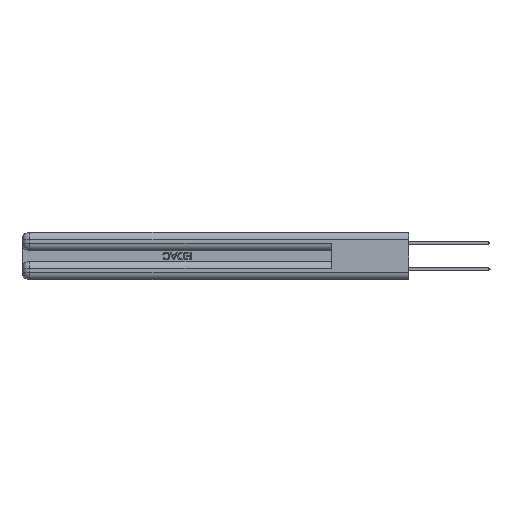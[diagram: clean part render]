
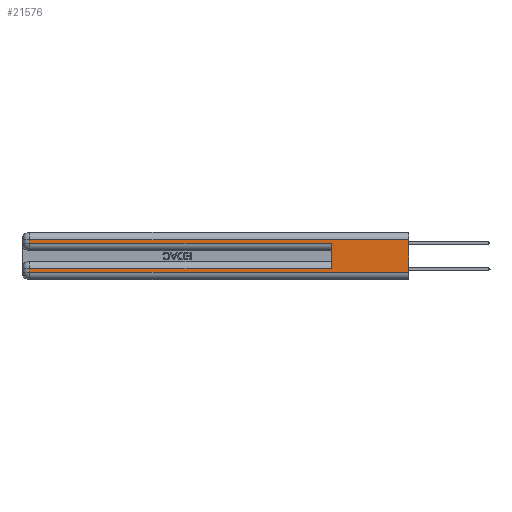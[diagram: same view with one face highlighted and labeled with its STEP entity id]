
A CAD part, left-side view. The second image highlights one B-rep face of the part: STEP entity #21576.
In plain terms, the highlighted planar face has unit normal (-1, 0, 0).
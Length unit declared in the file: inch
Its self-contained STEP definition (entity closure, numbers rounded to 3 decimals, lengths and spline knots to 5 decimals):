
#210 = AXIS2_PLACEMENT_3D ( 'NONE', #48010, #25254, #2502 ) ;
#254 = LINE ( 'NONE', #2577, #39509 ) ;
#1376 = LINE ( 'NONE', #38945, #48323 ) ;
#2502 = DIRECTION ( 'NONE',  ( 0., 0., -1. ) ) ;
#2577 = CARTESIAN_POINT ( 'NONE',  ( 0., 0., 0.31 ) ) ;
#2820 = CARTESIAN_POINT ( 'NONE',  ( 0., 2.94, 0.06 ) ) ;
#3358 = DIRECTION ( 'NONE',  ( 0., 0., 1. ) ) ;
#3640 = CARTESIAN_POINT ( 'NONE',  ( 0., 2.94, 0.085 ) ) ;
#4225 = VECTOR ( 'NONE', #24502, 39.37008 ) ;
#4384 = CARTESIAN_POINT ( 'NONE',  ( 0., 0., 0.31 ) ) ;
#7196 = EDGE_CURVE ( 'NONE', #16572, #26620, #23655, .T. ) ;
#8364 = CARTESIAN_POINT ( 'NONE',  ( 0., 2.94, 0.37 ) ) ;
#9181 = VECTOR ( 'NONE', #3358, 39.37008 ) ;
#9287 = ORIENTED_EDGE ( 'NONE', *, *, #15820, .F. ) ;
#10063 = DIRECTION ( 'NONE',  ( 0., 1., 0. ) ) ;
#10263 = EDGE_CURVE ( 'NONE', #26580, #30235, #36626, .T. ) ;
#11100 = ORIENTED_EDGE ( 'NONE', *, *, #7196, .T. ) ;
#12165 = CARTESIAN_POINT ( 'NONE',  ( 0., 0., 0.06 ) ) ;
#12477 = EDGE_CURVE ( 'NONE', #35726, #39090, #1376, .T. ) ;
#12844 = EDGE_CURVE ( 'NONE', #26620, #39090, #15602, .T. ) ;
#13586 = ORIENTED_EDGE ( 'NONE', *, *, #10263, .T. ) ;
#13839 = VERTEX_POINT ( 'NONE', #37634 ) ;
#14327 = LINE ( 'NONE', #39448, #4225 ) ;
#14745 = DIRECTION ( 'NONE',  ( 0., 1., 0. ) ) ;
#15009 = CARTESIAN_POINT ( 'NONE',  ( 0., 0.6, 0.145 ) ) ;
#15602 = LINE ( 'NONE', #12165, #48854 ) ;
#15779 = ORIENTED_EDGE ( 'NONE', *, *, #12477, .F. ) ;
#15820 = EDGE_CURVE ( 'NONE', #44674, #30235, #47198, .T. ) ;
#16572 = VERTEX_POINT ( 'NONE', #3640 ) ;
#18968 = EDGE_LOOP ( 'NONE', ( #15779, #25757, #38064, #13586, #9287, #26929, #11100, #25933 ) ) ;
#21217 = VECTOR ( 'NONE', #26744, 39.37008 ) ;
#21576 = ADVANCED_FACE ( 'NONE', ( #31222 ), #25100, .F. ) ;
#23655 = LINE ( 'NONE', #8364, #37308 ) ;
#24345 = DIRECTION ( 'NONE',  ( 0., 0., -1. ) ) ;
#24502 = DIRECTION ( 'NONE',  ( 0., 0., -1. ) ) ;
#25100 = PLANE ( 'NONE',  #210 ) ;
#25254 = DIRECTION ( 'NONE',  ( 1., 0., 0. ) ) ;
#25298 = VECTOR ( 'NONE', #14745, 39.37008 ) ;
#25757 = ORIENTED_EDGE ( 'NONE', *, *, #29008, .T. ) ;
#25933 = ORIENTED_EDGE ( 'NONE', *, *, #12844, .T. ) ;
#26580 = VERTEX_POINT ( 'NONE', #41015 ) ;
#26620 = VERTEX_POINT ( 'NONE', #2820 ) ;
#26744 = DIRECTION ( 'NONE',  ( 0., -1., 0. ) ) ;
#26929 = ORIENTED_EDGE ( 'NONE', *, *, #28510, .T. ) ;
#27068 = CARTESIAN_POINT ( 'NONE',  ( 0., 0., 0.285 ) ) ;
#27883 = CARTESIAN_POINT ( 'NONE',  ( 0., 0., 0.06 ) ) ;
#28510 = EDGE_CURVE ( 'NONE', #44674, #16572, #45503, .T. ) ;
#29008 = EDGE_CURVE ( 'NONE', #35726, #13839, #254, .T. ) ;
#30235 = VERTEX_POINT ( 'NONE', #38390 ) ;
#31222 = FACE_OUTER_BOUND ( 'NONE', #18968, .T. ) ;
#33185 = CARTESIAN_POINT ( 'NONE',  ( 0., 0., 0.085 ) ) ;
#34851 = DIRECTION ( 'NONE',  ( 0., 0., -1. ) ) ;
#35726 = VERTEX_POINT ( 'NONE', #4384 ) ;
#36626 = LINE ( 'NONE', #27068, #21217 ) ;
#37308 = VECTOR ( 'NONE', #34851, 39.37008 ) ;
#37634 = CARTESIAN_POINT ( 'NONE',  ( 0., 2.94, 0.31 ) ) ;
#38064 = ORIENTED_EDGE ( 'NONE', *, *, #48570, .T. ) ;
#38390 = CARTESIAN_POINT ( 'NONE',  ( 0., 0.6, 0.285 ) ) ;
#38945 = CARTESIAN_POINT ( 'NONE',  ( 0., 0., 0.37 ) ) ;
#39090 = VERTEX_POINT ( 'NONE', #27883 ) ;
#39448 = CARTESIAN_POINT ( 'NONE',  ( 0., 2.94, 0.37 ) ) ;
#39509 = VECTOR ( 'NONE', #10063, 39.37008 ) ;
#40763 = CARTESIAN_POINT ( 'NONE',  ( 0., 0.6, 0.085 ) ) ;
#41015 = CARTESIAN_POINT ( 'NONE',  ( 0., 2.94, 0.285 ) ) ;
#44674 = VERTEX_POINT ( 'NONE', #40763 ) ;
#45503 = LINE ( 'NONE', #33185, #25298 ) ;
#46215 = DIRECTION ( 'NONE',  ( 0., -1., 0. ) ) ;
#47198 = LINE ( 'NONE', #15009, #9181 ) ;
#48010 = CARTESIAN_POINT ( 'NONE',  ( 0., 0., 0.37 ) ) ;
#48323 = VECTOR ( 'NONE', #24345, 39.37008 ) ;
#48570 = EDGE_CURVE ( 'NONE', #13839, #26580, #14327, .T. ) ;
#48854 = VECTOR ( 'NONE', #46215, 39.37008 ) ;
